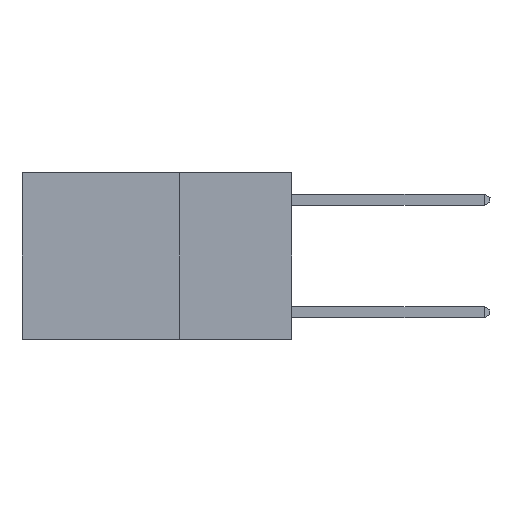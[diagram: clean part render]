
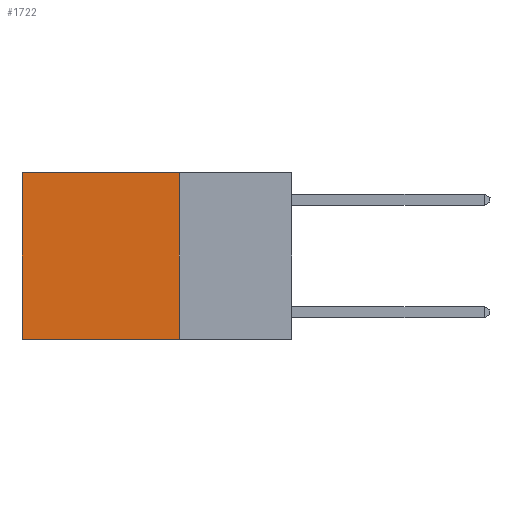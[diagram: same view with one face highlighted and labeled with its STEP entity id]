
A CAD part, left-side view. The second image highlights one B-rep face of the part: STEP entity #1722.
In plain terms, the highlighted planar face has unit normal (-1, 0, 0).
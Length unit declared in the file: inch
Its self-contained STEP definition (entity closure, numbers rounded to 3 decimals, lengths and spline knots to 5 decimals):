
#480 = VECTOR ( 'NONE', #4374, 39.37008 ) ;
#744 = CARTESIAN_POINT ( 'NONE',  ( 0.2625, 0.6, -0.37 ) ) ;
#1414 = DIRECTION ( 'NONE',  ( 0., 0., -1. ) ) ;
#1722 = ADVANCED_FACE ( 'NONE', ( #19462 ), #22561, .F. ) ;
#2354 = ORIENTED_EDGE ( 'NONE', *, *, #11258, .T. ) ;
#4374 = DIRECTION ( 'NONE',  ( 0., 0., -1. ) ) ;
#5040 = CARTESIAN_POINT ( 'NONE',  ( 0.2625, 0.6, 0. ) ) ;
#5857 = ORIENTED_EDGE ( 'NONE', *, *, #18365, .F. ) ;
#6285 = DIRECTION ( 'NONE',  ( 0., 0., -1. ) ) ;
#6432 = LINE ( 'NONE', #6605, #20678 ) ;
#6605 = CARTESIAN_POINT ( 'NONE',  ( 0.2625, 0.25, 0. ) ) ;
#7099 = VECTOR ( 'NONE', #8571, 39.37008 ) ;
#7795 = AXIS2_PLACEMENT_3D ( 'NONE', #11359, #11435, #6285 ) ;
#7991 = CARTESIAN_POINT ( 'NONE',  ( 0.2625, 0.25, 0. ) ) ;
#8571 = DIRECTION ( 'NONE',  ( 0., 1., 0. ) ) ;
#9646 = ORIENTED_EDGE ( 'NONE', *, *, #24154, .F. ) ;
#10249 = VERTEX_POINT ( 'NONE', #18554 ) ;
#10679 = VERTEX_POINT ( 'NONE', #21778 ) ;
#11258 = EDGE_CURVE ( 'NONE', #10679, #15950, #6432, .T. ) ;
#11359 = CARTESIAN_POINT ( 'NONE',  ( 0.2625, 0.25, 0. ) ) ;
#11435 = DIRECTION ( 'NONE',  ( 1., 0., 0. ) ) ;
#11483 = LINE ( 'NONE', #19731, #7099 ) ;
#14061 = LINE ( 'NONE', #18312, #22725 ) ;
#15950 = VERTEX_POINT ( 'NONE', #5040 ) ;
#16043 = EDGE_CURVE ( 'NONE', #15950, #20762, #14061, .T. ) ;
#18312 = CARTESIAN_POINT ( 'NONE',  ( 0.2625, 0.6, 0. ) ) ;
#18365 = EDGE_CURVE ( 'NONE', #10249, #20762, #11483, .T. ) ;
#18554 = CARTESIAN_POINT ( 'NONE',  ( 0.2625, 0.25, -0.37 ) ) ;
#19462 = FACE_OUTER_BOUND ( 'NONE', #21920, .T. ) ;
#19647 = DIRECTION ( 'NONE',  ( 0., 1., 0. ) ) ;
#19731 = CARTESIAN_POINT ( 'NONE',  ( 0.2625, 0.25, -0.37 ) ) ;
#20127 = ORIENTED_EDGE ( 'NONE', *, *, #16043, .T. ) ;
#20678 = VECTOR ( 'NONE', #19647, 39.37008 ) ;
#20762 = VERTEX_POINT ( 'NONE', #744 ) ;
#21092 = LINE ( 'NONE', #7991, #480 ) ;
#21778 = CARTESIAN_POINT ( 'NONE',  ( 0.2625, 0.25, 0. ) ) ;
#21920 = EDGE_LOOP ( 'NONE', ( #20127, #5857, #9646, #2354 ) ) ;
#22561 = PLANE ( 'NONE',  #7795 ) ;
#22725 = VECTOR ( 'NONE', #1414, 39.37008 ) ;
#24154 = EDGE_CURVE ( 'NONE', #10679, #10249, #21092, .T. ) ;
